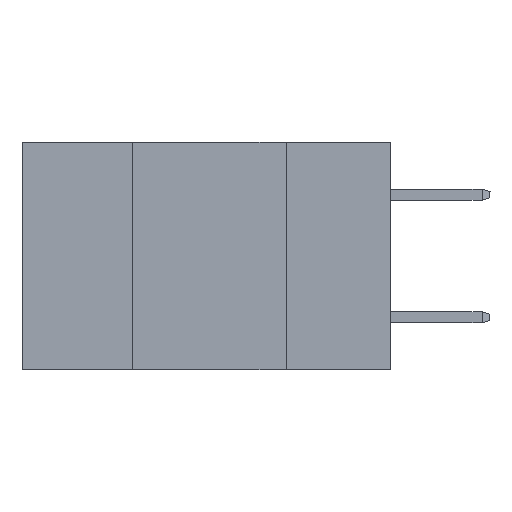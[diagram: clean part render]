
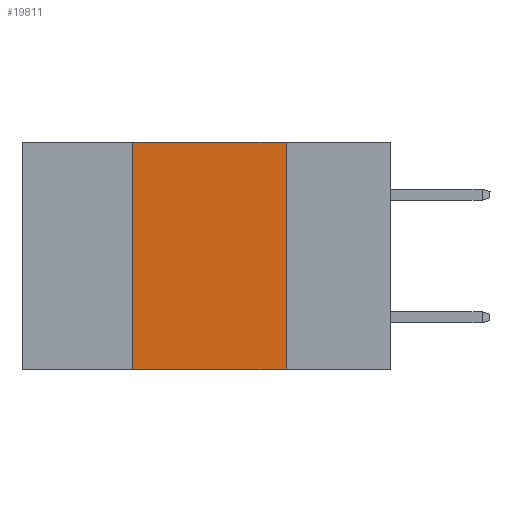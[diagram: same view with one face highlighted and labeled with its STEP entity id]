
A CAD part, left-side view. The second image highlights one B-rep face of the part: STEP entity #19811.
In plain terms, the highlighted planar face has unit normal (-1, 0, 0).
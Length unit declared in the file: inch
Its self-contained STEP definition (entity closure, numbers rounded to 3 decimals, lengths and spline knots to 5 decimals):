
#7 = CARTESIAN_POINT ( 'NONE',  ( 0., 0.17, -0.37 ) ) ;
#130 = CARTESIAN_POINT ( 'NONE',  ( 0., 0.6, 0. ) ) ;
#541 = EDGE_CURVE ( 'NONE', #13231, #3416, #35000, .T. ) ;
#1704 = CARTESIAN_POINT ( 'NONE',  ( 0., 0.42, -0.37 ) ) ;
#1739 = DIRECTION ( 'NONE',  ( 0., 0., -1. ) ) ;
#3227 = CARTESIAN_POINT ( 'NONE',  ( 0., 0.17, 0. ) ) ;
#3416 = VERTEX_POINT ( 'NONE', #7 ) ;
#3428 = FACE_OUTER_BOUND ( 'NONE', #29722, .T. ) ;
#7575 = DIRECTION ( 'NONE',  ( 0., 0., 1. ) ) ;
#9885 = VERTEX_POINT ( 'NONE', #33292 ) ;
#11674 = VECTOR ( 'NONE', #1739, 39.37008 ) ;
#13231 = VERTEX_POINT ( 'NONE', #3227 ) ;
#13996 = DIRECTION ( 'NONE',  ( 1., 0., 0. ) ) ;
#15700 = EDGE_CURVE ( 'NONE', #30594, #3416, #33611, .T. ) ;
#16757 = CARTESIAN_POINT ( 'NONE',  ( 0., 0.42, 0. ) ) ;
#18152 = AXIS2_PLACEMENT_3D ( 'NONE', #27511, #13996, #21540 ) ;
#19811 = ADVANCED_FACE ( 'NONE', ( #3428 ), #33627, .F. ) ;
#20136 = LINE ( 'NONE', #130, #34375 ) ;
#20864 = VECTOR ( 'NONE', #7575, 39.37008 ) ;
#21540 = DIRECTION ( 'NONE',  ( 0., 0., -1. ) ) ;
#23119 = EDGE_CURVE ( 'NONE', #30594, #9885, #36997, .T. ) ;
#23267 = CARTESIAN_POINT ( 'NONE',  ( 0., 0.17, 0. ) ) ;
#25583 = VECTOR ( 'NONE', #30379, 39.37008 ) ;
#27075 = EDGE_CURVE ( 'NONE', #9885, #13231, #20136, .T. ) ;
#27187 = CARTESIAN_POINT ( 'NONE',  ( 0., 0.6, -0.37 ) ) ;
#27511 = CARTESIAN_POINT ( 'NONE',  ( 0., 0.6, 0. ) ) ;
#29722 = EDGE_LOOP ( 'NONE', ( #37160, #34531, #30069, #35125 ) ) ;
#30069 = ORIENTED_EDGE ( 'NONE', *, *, #23119, .F. ) ;
#30379 = DIRECTION ( 'NONE',  ( 0., -1., 0. ) ) ;
#30594 = VERTEX_POINT ( 'NONE', #1704 ) ;
#30850 = DIRECTION ( 'NONE',  ( 0., -1., 0. ) ) ;
#33292 = CARTESIAN_POINT ( 'NONE',  ( 0., 0.42, 0. ) ) ;
#33611 = LINE ( 'NONE', #27187, #25583 ) ;
#33627 = PLANE ( 'NONE',  #18152 ) ;
#34375 = VECTOR ( 'NONE', #30850, 39.37008 ) ;
#34531 = ORIENTED_EDGE ( 'NONE', *, *, #27075, .F. ) ;
#35000 = LINE ( 'NONE', #23267, #11674 ) ;
#35125 = ORIENTED_EDGE ( 'NONE', *, *, #15700, .T. ) ;
#36997 = LINE ( 'NONE', #16757, #20864 ) ;
#37160 = ORIENTED_EDGE ( 'NONE', *, *, #541, .F. ) ;
